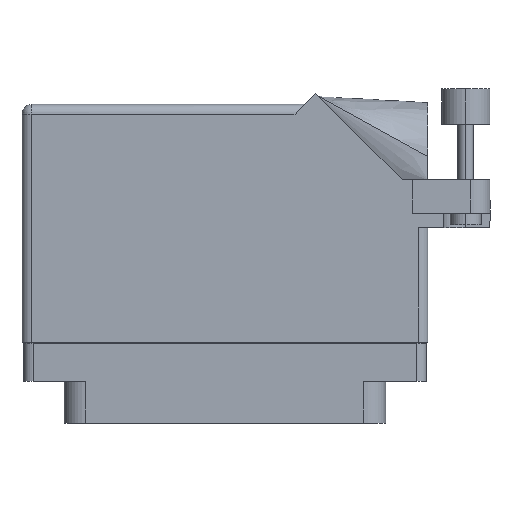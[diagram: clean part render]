
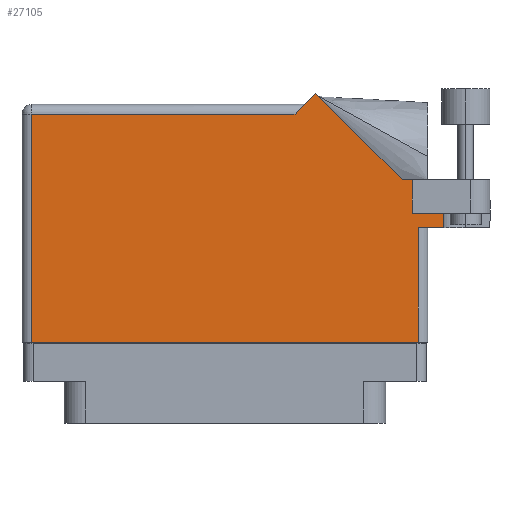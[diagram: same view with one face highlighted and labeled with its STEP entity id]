
A CAD part, front view. The second image highlights one B-rep face of the part: STEP entity #27105.
In plain terms, the highlighted face is planar.
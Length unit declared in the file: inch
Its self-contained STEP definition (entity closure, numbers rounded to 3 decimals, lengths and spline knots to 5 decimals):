
#93 = VECTOR ( 'NONE', #30073, 39.37008 ) ;
#356 = CARTESIAN_POINT ( 'NONE',  ( -1.244, -0.1, 0.455 ) ) ;
#521 = EDGE_CURVE ( 'NONE', #17942, #14847, #10103, .T. ) ;
#977 = EDGE_CURVE ( 'NONE', #26052, #14847, #21117, .T. ) ;
#1134 = EDGE_CURVE ( 'NONE', #47553, #39237, #18806, .T. ) ;
#1775 = CARTESIAN_POINT ( 'NONE',  ( 1.206, 0.944, 0.455 ) ) ;
#1823 = DIRECTION ( 'NONE',  ( 0., 0., -1. ) ) ;
#2508 = VERTEX_POINT ( 'NONE', #37344 ) ;
#2864 = CARTESIAN_POINT ( 'NONE',  ( 1.244, 0.637, 0.455 ) ) ;
#2870 = ORIENTED_EDGE ( 'NONE', *, *, #521, .F. ) ;
#4098 = LINE ( 'NONE', #34278, #19310 ) ;
#4110 = EDGE_CURVE ( 'NONE', #27635, #47589, #34414, .T. ) ;
#4280 = ORIENTED_EDGE ( 'NONE', *, *, #8718, .F. ) ;
#4723 = DIRECTION ( 'NONE',  ( 0., -1., 0. ) ) ;
#5095 = EDGE_LOOP ( 'NONE', ( #33827, #17151, #23563, #2870, #4280, #29194, #30491, #39259, #14896, #21918, #35846 ) ) ;
#5899 = PLANE ( 'NONE',  #17780 ) ;
#6789 = DIRECTION ( 'NONE',  ( 0., 1., 0. ) ) ;
#8718 = EDGE_CURVE ( 'NONE', #27635, #17942, #4098, .T. ) ;
#8780 = CARTESIAN_POINT ( 'NONE',  ( 1.14042, 0.944, 0.455 ) ) ;
#8826 = VECTOR ( 'NONE', #31608, 39.37008 ) ;
#8934 = VECTOR ( 'NONE', #15306, 39.37008 ) ;
#9151 = CARTESIAN_POINT ( 'NONE',  ( -1.306, 1.43, 0.455 ) ) ;
#9671 = CARTESIAN_POINT ( 'NONE',  ( -1.306, -0.1, 0.455 ) ) ;
#10103 = LINE ( 'NONE', #45231, #8934 ) ;
#10202 = EDGE_CURVE ( 'NONE', #47589, #44054, #36917, .T. ) ;
#11369 = VECTOR ( 'NONE', #46361, 39.37008 ) ;
#12878 = EDGE_CURVE ( 'NONE', #2508, #19754, #15758, .T. ) ;
#13252 = DIRECTION ( 'NONE',  ( 0., 1., 0. ) ) ;
#14847 = VERTEX_POINT ( 'NONE', #22917 ) ;
#14896 = ORIENTED_EDGE ( 'NONE', *, *, #1134, .T. ) ;
#15306 = DIRECTION ( 'NONE',  ( 0., -1., 0. ) ) ;
#15723 = CARTESIAN_POINT ( 'NONE',  ( 1.306, 0.637, 0.455 ) ) ;
#15758 = LINE ( 'NONE', #356, #41194 ) ;
#15864 = DIRECTION ( 'NONE',  ( 1., 0., 0. ) ) ;
#15883 = VECTOR ( 'NONE', #39953, 39.37008 ) ;
#16929 = CARTESIAN_POINT ( 'NONE',  ( 1.244, -0.1, 0.455 ) ) ;
#17151 = ORIENTED_EDGE ( 'NONE', *, *, #20323, .T. ) ;
#17780 = AXIS2_PLACEMENT_3D ( 'NONE', #9151, #1823, #23964 ) ;
#17942 = VERTEX_POINT ( 'NONE', #35286 ) ;
#18186 = LINE ( 'NONE', #9671, #32649 ) ;
#18210 = VERTEX_POINT ( 'NONE', #16929 ) ;
#18806 = LINE ( 'NONE', #24099, #15883 ) ;
#19093 = CARTESIAN_POINT ( 'NONE',  ( 1.244, 0.637, 0.455 ) ) ;
#19310 = VECTOR ( 'NONE', #15864, 39.37008 ) ;
#19754 = VERTEX_POINT ( 'NONE', #38164 ) ;
#20323 = EDGE_CURVE ( 'NONE', #18210, #26052, #38700, .T. ) ;
#20594 = CARTESIAN_POINT ( 'NONE',  ( 1.206, 0.731, 0.455 ) ) ;
#21117 = LINE ( 'NONE', #15723, #93 ) ;
#21918 = ORIENTED_EDGE ( 'NONE', *, *, #46923, .T. ) ;
#22917 = CARTESIAN_POINT ( 'NONE',  ( 1.4075, 0.637, 0.455 ) ) ;
#23563 = ORIENTED_EDGE ( 'NONE', *, *, #977, .T. ) ;
#23964 = DIRECTION ( 'NONE',  ( -1., 0., 0. ) ) ;
#24099 = CARTESIAN_POINT ( 'NONE',  ( 0.513, 1.43, 0.455 ) ) ;
#25618 = CARTESIAN_POINT ( 'NONE',  ( 1.14042, 0.944, 0.455 ) ) ;
#26052 = VERTEX_POINT ( 'NONE', #19093 ) ;
#27105 = ADVANCED_FACE ( 'NONE', ( #29367 ), #5899, .F. ) ;
#27455 = CARTESIAN_POINT ( 'NONE',  ( 0.58371, 1.50071, 0.455 ) ) ;
#27635 = VERTEX_POINT ( 'NONE', #37086 ) ;
#28834 = VECTOR ( 'NONE', #6789, 39.37008 ) ;
#29186 = VECTOR ( 'NONE', #13252, 39.37008 ) ;
#29194 = ORIENTED_EDGE ( 'NONE', *, *, #4110, .T. ) ;
#29318 = VECTOR ( 'NONE', #34142, 39.37008 ) ;
#29367 = FACE_OUTER_BOUND ( 'NONE', #5095, .T. ) ;
#30073 = DIRECTION ( 'NONE',  ( 1., 0., 0. ) ) ;
#30491 = ORIENTED_EDGE ( 'NONE', *, *, #10202, .T. ) ;
#30737 = DIRECTION ( 'NONE',  ( 1., 0., 0. ) ) ;
#31608 = DIRECTION ( 'NONE',  ( -1., 0., 0. ) ) ;
#32649 = VECTOR ( 'NONE', #30737, 39.37008 ) ;
#33827 = ORIENTED_EDGE ( 'NONE', *, *, #47318, .T. ) ;
#34142 = DIRECTION ( 'NONE',  ( -0.707, 0.707, 0. ) ) ;
#34278 = CARTESIAN_POINT ( 'NONE',  ( 1.206, 0.731, 0.455 ) ) ;
#34414 = LINE ( 'NONE', #20594, #29186 ) ;
#35286 = CARTESIAN_POINT ( 'NONE',  ( 1.4075, 0.731, 0.455 ) ) ;
#35846 = ORIENTED_EDGE ( 'NONE', *, *, #12878, .T. ) ;
#36917 = LINE ( 'NONE', #46197, #11369 ) ;
#37086 = CARTESIAN_POINT ( 'NONE',  ( 1.206, 0.731, 0.455 ) ) ;
#37344 = CARTESIAN_POINT ( 'NONE',  ( -1.244, 1.368, 0.455 ) ) ;
#38164 = CARTESIAN_POINT ( 'NONE',  ( -1.244, -0.1, 0.455 ) ) ;
#38384 = CARTESIAN_POINT ( 'NONE',  ( 0.451, 1.368, 0.455 ) ) ;
#38700 = LINE ( 'NONE', #2864, #28834 ) ;
#39207 = LINE ( 'NONE', #8780, #29318 ) ;
#39237 = VERTEX_POINT ( 'NONE', #38384 ) ;
#39249 = CARTESIAN_POINT ( 'NONE',  ( -1.306, 1.368, 0.455 ) ) ;
#39259 = ORIENTED_EDGE ( 'NONE', *, *, #44188, .T. ) ;
#39953 = DIRECTION ( 'NONE',  ( -0.707, -0.707, 0. ) ) ;
#40784 = LINE ( 'NONE', #39249, #8826 ) ;
#41194 = VECTOR ( 'NONE', #4723, 39.37008 ) ;
#44054 = VERTEX_POINT ( 'NONE', #25618 ) ;
#44188 = EDGE_CURVE ( 'NONE', #44054, #47553, #39207, .T. ) ;
#45231 = CARTESIAN_POINT ( 'NONE',  ( 1.4075, 1.06177, 0.455 ) ) ;
#46197 = CARTESIAN_POINT ( 'NONE',  ( 1.706, 0.944, 0.455 ) ) ;
#46361 = DIRECTION ( 'NONE',  ( -1., 0., 0. ) ) ;
#46923 = EDGE_CURVE ( 'NONE', #39237, #2508, #40784, .T. ) ;
#47318 = EDGE_CURVE ( 'NONE', #19754, #18210, #18186, .T. ) ;
#47553 = VERTEX_POINT ( 'NONE', #27455 ) ;
#47589 = VERTEX_POINT ( 'NONE', #1775 ) ;
